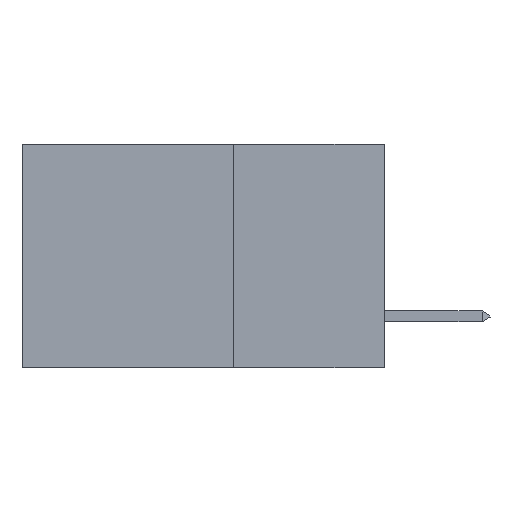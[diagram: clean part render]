
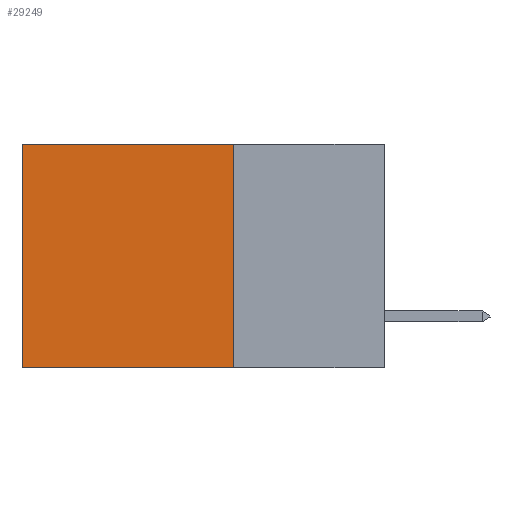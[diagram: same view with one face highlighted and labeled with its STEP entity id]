
A CAD part, left-side view. The second image highlights one B-rep face of the part: STEP entity #29249.
In plain terms, the highlighted planar face has unit normal (-1, 0, 0).
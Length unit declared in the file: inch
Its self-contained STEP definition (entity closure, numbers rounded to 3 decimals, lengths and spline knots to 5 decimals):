
#130 = CARTESIAN_POINT ( 'NONE',  ( 0.2875, 0.6, 0. ) ) ;
#544 = VECTOR ( 'NONE', #46663, 39.37008 ) ;
#1063 = EDGE_CURVE ( 'NONE', #40602, #32673, #4015, .T. ) ;
#4015 = LINE ( 'NONE', #30715, #21709 ) ;
#4093 = LINE ( 'NONE', #130, #47865 ) ;
#6591 = CARTESIAN_POINT ( 'NONE',  ( 0.2875, 0.25, 0. ) ) ;
#7057 = DIRECTION ( 'NONE',  ( 0., 1., 0. ) ) ;
#10642 = LINE ( 'NONE', #31629, #544 ) ;
#11645 = EDGE_CURVE ( 'NONE', #40602, #31796, #32465, .T. ) ;
#14213 = ORIENTED_EDGE ( 'NONE', *, *, #32660, .F. ) ;
#15728 = CARTESIAN_POINT ( 'NONE',  ( 0.2875, 0.6, 0. ) ) ;
#16432 = CARTESIAN_POINT ( 'NONE',  ( 0.2875, 0.25, -0.37 ) ) ;
#17113 = VECTOR ( 'NONE', #7057, 39.37008 ) ;
#17480 = PLANE ( 'NONE',  #29102 ) ;
#18159 = ORIENTED_EDGE ( 'NONE', *, *, #18520, .T. ) ;
#18433 = CARTESIAN_POINT ( 'NONE',  ( 0.2875, 0.25, 0. ) ) ;
#18520 = EDGE_CURVE ( 'NONE', #31796, #35052, #4093, .T. ) ;
#21709 = VECTOR ( 'NONE', #42274, 39.37008 ) ;
#24380 = ORIENTED_EDGE ( 'NONE', *, *, #1063, .F. ) ;
#24883 = DIRECTION ( 'NONE',  ( 0., 0., -1. ) ) ;
#26383 = FACE_OUTER_BOUND ( 'NONE', #39409, .T. ) ;
#29102 = AXIS2_PLACEMENT_3D ( 'NONE', #6591, #40411, #24883 ) ;
#29249 = ADVANCED_FACE ( 'NONE', ( #26383 ), #17480, .F. ) ;
#30715 = CARTESIAN_POINT ( 'NONE',  ( 0.2875, 0.25, 0. ) ) ;
#30864 = DIRECTION ( 'NONE',  ( 0., 0., -1. ) ) ;
#31629 = CARTESIAN_POINT ( 'NONE',  ( 0.2875, 0.25, -0.37 ) ) ;
#31796 = VERTEX_POINT ( 'NONE', #15728 ) ;
#32465 = LINE ( 'NONE', #18433, #17113 ) ;
#32660 = EDGE_CURVE ( 'NONE', #32673, #35052, #10642, .T. ) ;
#32673 = VERTEX_POINT ( 'NONE', #16432 ) ;
#34469 = CARTESIAN_POINT ( 'NONE',  ( 0.2875, 0.25, 0. ) ) ;
#35052 = VERTEX_POINT ( 'NONE', #42398 ) ;
#39239 = ORIENTED_EDGE ( 'NONE', *, *, #11645, .T. ) ;
#39409 = EDGE_LOOP ( 'NONE', ( #18159, #14213, #24380, #39239 ) ) ;
#40411 = DIRECTION ( 'NONE',  ( 1., 0., 0. ) ) ;
#40602 = VERTEX_POINT ( 'NONE', #34469 ) ;
#42274 = DIRECTION ( 'NONE',  ( 0., 0., -1. ) ) ;
#42398 = CARTESIAN_POINT ( 'NONE',  ( 0.2875, 0.6, -0.37 ) ) ;
#46663 = DIRECTION ( 'NONE',  ( 0., 1., 0. ) ) ;
#47865 = VECTOR ( 'NONE', #30864, 39.37008 ) ;
